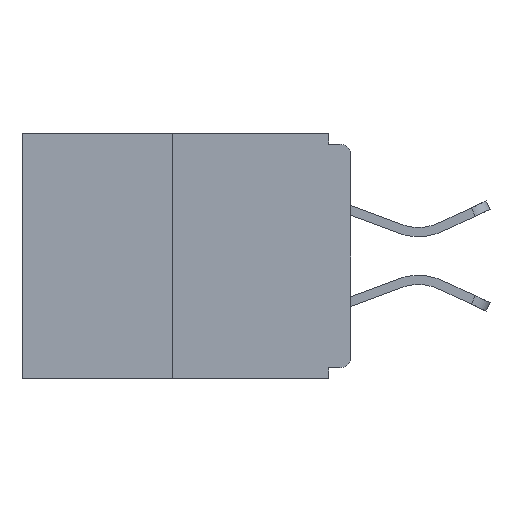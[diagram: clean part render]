
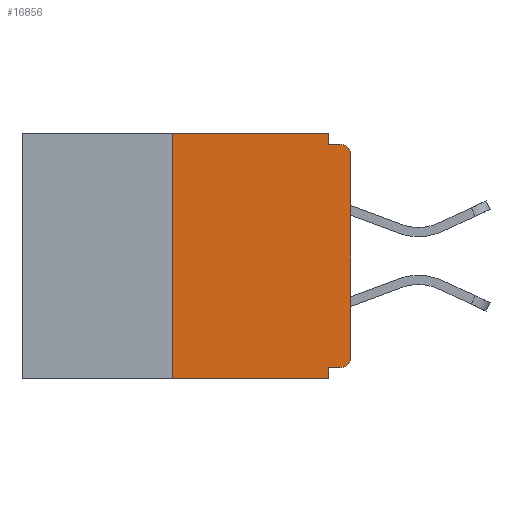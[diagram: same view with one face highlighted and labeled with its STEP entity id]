
A CAD part, left-side view. The second image highlights one B-rep face of the part: STEP entity #16856.
In plain terms, the highlighted planar face has unit normal (-1, 0, 0).
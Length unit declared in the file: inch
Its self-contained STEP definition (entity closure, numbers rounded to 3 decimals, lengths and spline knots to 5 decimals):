
#288 = DIRECTION ( 'NONE',  ( 0., 0., -1. ) ) ;
#467 = CARTESIAN_POINT ( 'NONE',  ( 0., 0., -0.328 ) ) ;
#559 = CARTESIAN_POINT ( 'NONE',  ( 0., 0.46, 0. ) ) ;
#607 = VECTOR ( 'NONE', #15359, 39.37008 ) ;
#960 = DIRECTION ( 'NONE',  ( 0., -1., 0. ) ) ;
#1232 = CARTESIAN_POINT ( 'NONE',  ( 0., 0.015, -0.313 ) ) ;
#2477 = CARTESIAN_POINT ( 'NONE',  ( 0., 0.015, -0.03 ) ) ;
#2504 = CARTESIAN_POINT ( 'NONE',  ( 0., 0.015, -0.015 ) ) ;
#2714 = CARTESIAN_POINT ( 'NONE',  ( 0., 0.46, -0.343 ) ) ;
#3118 = ORIENTED_EDGE ( 'NONE', *, *, #3874, .T. ) ;
#3243 = CARTESIAN_POINT ( 'NONE',  ( 0., 0.031, -0.343 ) ) ;
#3449 = DIRECTION ( 'NONE',  ( 0., 0., -1. ) ) ;
#3874 = EDGE_CURVE ( 'NONE', #27330, #26747, #17457, .T. ) ;
#4144 = EDGE_CURVE ( 'NONE', #27330, #12524, #12198, .T. ) ;
#4488 = CARTESIAN_POINT ( 'NONE',  ( 0., 0.015, -0.328 ) ) ;
#4695 = VECTOR ( 'NONE', #23200, 39.37008 ) ;
#5282 = LINE ( 'NONE', #2714, #8799 ) ;
#6175 = CARTESIAN_POINT ( 'NONE',  ( 0., 0.46, 0. ) ) ;
#6611 = VERTEX_POINT ( 'NONE', #2504 ) ;
#6673 = ORIENTED_EDGE ( 'NONE', *, *, #24113, .F. ) ;
#6989 = CIRCLE ( 'NONE', #17891, 0.015 ) ;
#7074 = DIRECTION ( 'NONE',  ( 0., 1., 0. ) ) ;
#7194 = EDGE_CURVE ( 'NONE', #24844, #16925, #24563, .T. ) ;
#8324 = CARTESIAN_POINT ( 'NONE',  ( 0., 0., 0. ) ) ;
#8684 = CARTESIAN_POINT ( 'NONE',  ( 0., 0., -0.03 ) ) ;
#8799 = VECTOR ( 'NONE', #22463, 39.37008 ) ;
#8927 = EDGE_CURVE ( 'NONE', #12524, #23636, #17642, .T. ) ;
#10134 = EDGE_LOOP ( 'NONE', ( #6673, #20102, #22742, #15423, #22614, #3118, #24139, #18462, #17083, #22780 ) ) ;
#10249 = CARTESIAN_POINT ( 'NONE',  ( 0., 0.031, 0. ) ) ;
#10444 = DIRECTION ( 'NONE',  ( 0., 0., -1. ) ) ;
#10512 = VECTOR ( 'NONE', #12769, 39.37008 ) ;
#10549 = DIRECTION ( 'NONE',  ( 0., 0., 1. ) ) ;
#11173 = LINE ( 'NONE', #559, #23410 ) ;
#11483 = EDGE_CURVE ( 'NONE', #27646, #15292, #19281, .T. ) ;
#11504 = CARTESIAN_POINT ( 'NONE',  ( 0., 0.25, -0.343 ) ) ;
#12198 = LINE ( 'NONE', #467, #15672 ) ;
#12524 = VERTEX_POINT ( 'NONE', #18653 ) ;
#12760 = VECTOR ( 'NONE', #288, 39.37008 ) ;
#12769 = DIRECTION ( 'NONE',  ( 0., 0., 1. ) ) ;
#13107 = CARTESIAN_POINT ( 'NONE',  ( 0., 0.25, 0. ) ) ;
#14556 = LINE ( 'NONE', #19951, #607 ) ;
#15292 = VERTEX_POINT ( 'NONE', #13107 ) ;
#15359 = DIRECTION ( 'NONE',  ( 0., -1., 0. ) ) ;
#15423 = ORIENTED_EDGE ( 'NONE', *, *, #8927, .F. ) ;
#15672 = VECTOR ( 'NONE', #7074, 39.37008 ) ;
#15978 = CARTESIAN_POINT ( 'NONE',  ( 0., 0.031, 0. ) ) ;
#16806 = DIRECTION ( 'NONE',  ( -1., 0., 0. ) ) ;
#16856 = ADVANCED_FACE ( 'NONE', ( #18965 ), #19256, .F. ) ;
#16893 = EDGE_CURVE ( 'NONE', #26747, #26102, #24150, .T. ) ;
#16925 = VERTEX_POINT ( 'NONE', #26411 ) ;
#17083 = ORIENTED_EDGE ( 'NONE', *, *, #26508, .F. ) ;
#17457 = CIRCLE ( 'NONE', #21659, 0.015 ) ;
#17513 = EDGE_CURVE ( 'NONE', #27646, #23636, #5282, .T. ) ;
#17642 = LINE ( 'NONE', #3243, #4695 ) ;
#17891 = AXIS2_PLACEMENT_3D ( 'NONE', #2477, #20309, #22523 ) ;
#18462 = ORIENTED_EDGE ( 'NONE', *, *, #18688, .T. ) ;
#18653 = CARTESIAN_POINT ( 'NONE',  ( 0., 0.031, -0.328 ) ) ;
#18688 = EDGE_CURVE ( 'NONE', #26102, #6611, #6989, .T. ) ;
#18965 = FACE_OUTER_BOUND ( 'NONE', #10134, .T. ) ;
#19256 = PLANE ( 'NONE',  #24713 ) ;
#19281 = LINE ( 'NONE', #21633, #10512 ) ;
#19652 = VECTOR ( 'NONE', #10549, 39.37008 ) ;
#19951 = CARTESIAN_POINT ( 'NONE',  ( 0., 0., -0.015 ) ) ;
#20102 = ORIENTED_EDGE ( 'NONE', *, *, #11483, .F. ) ;
#20305 = CARTESIAN_POINT ( 'NONE',  ( 0., 0.031, -0.343 ) ) ;
#20309 = DIRECTION ( 'NONE',  ( -1., 0., 0. ) ) ;
#21633 = CARTESIAN_POINT ( 'NONE',  ( 0., 0.25, 0. ) ) ;
#21659 = AXIS2_PLACEMENT_3D ( 'NONE', #1232, #16806, #3449 ) ;
#22463 = DIRECTION ( 'NONE',  ( 0., -1., 0. ) ) ;
#22523 = DIRECTION ( 'NONE',  ( 0., 0., -1. ) ) ;
#22614 = ORIENTED_EDGE ( 'NONE', *, *, #4144, .F. ) ;
#22742 = ORIENTED_EDGE ( 'NONE', *, *, #17513, .T. ) ;
#22780 = ORIENTED_EDGE ( 'NONE', *, *, #7194, .F. ) ;
#23200 = DIRECTION ( 'NONE',  ( 0., 0., -1. ) ) ;
#23229 = CARTESIAN_POINT ( 'NONE',  ( 0., 0., -0.313 ) ) ;
#23410 = VECTOR ( 'NONE', #960, 39.37008 ) ;
#23636 = VERTEX_POINT ( 'NONE', #20305 ) ;
#23812 = DIRECTION ( 'NONE',  ( 1., 0., 0. ) ) ;
#24113 = EDGE_CURVE ( 'NONE', #15292, #24844, #11173, .T. ) ;
#24139 = ORIENTED_EDGE ( 'NONE', *, *, #16893, .T. ) ;
#24150 = LINE ( 'NONE', #8324, #19652 ) ;
#24563 = LINE ( 'NONE', #15978, #12760 ) ;
#24713 = AXIS2_PLACEMENT_3D ( 'NONE', #6175, #23812, #10444 ) ;
#24844 = VERTEX_POINT ( 'NONE', #10249 ) ;
#26102 = VERTEX_POINT ( 'NONE', #8684 ) ;
#26411 = CARTESIAN_POINT ( 'NONE',  ( 0., 0.031, -0.015 ) ) ;
#26508 = EDGE_CURVE ( 'NONE', #16925, #6611, #14556, .T. ) ;
#26747 = VERTEX_POINT ( 'NONE', #23229 ) ;
#27330 = VERTEX_POINT ( 'NONE', #4488 ) ;
#27646 = VERTEX_POINT ( 'NONE', #11504 ) ;
